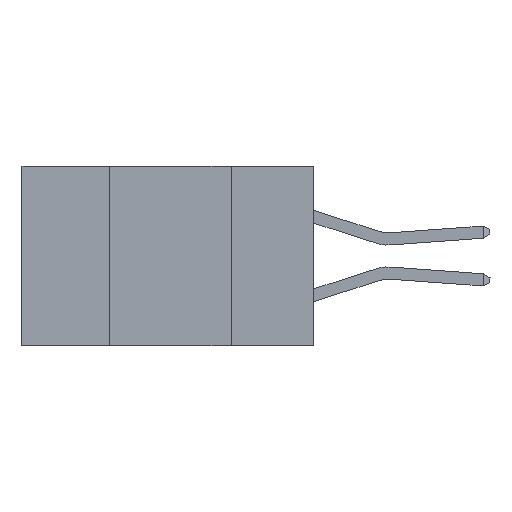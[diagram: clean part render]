
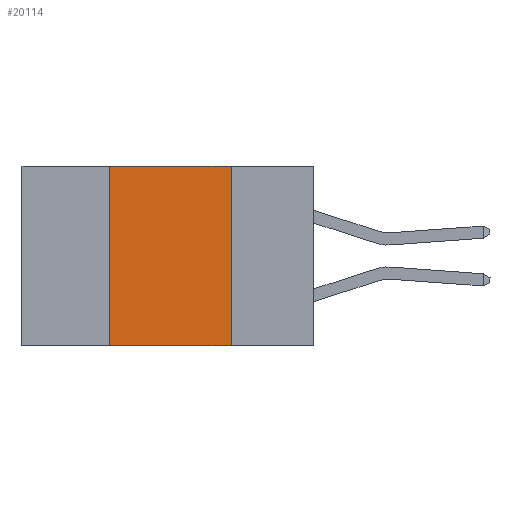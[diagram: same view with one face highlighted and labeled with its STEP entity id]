
A CAD part, left-side view. The second image highlights one B-rep face of the part: STEP entity #20114.
In plain terms, the highlighted planar face has unit normal (-1, 0, 0).
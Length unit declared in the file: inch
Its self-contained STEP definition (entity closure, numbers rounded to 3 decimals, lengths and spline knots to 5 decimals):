
#667 = CARTESIAN_POINT ( 'NONE',  ( 0., 0.17, 0. ) ) ;
#1285 = LINE ( 'NONE', #8244, #15098 ) ;
#1600 = DIRECTION ( 'NONE',  ( 0., 0., 1. ) ) ;
#1718 = ORIENTED_EDGE ( 'NONE', *, *, #7390, .T. ) ;
#2629 = VECTOR ( 'NONE', #1600, 39.37008 ) ;
#2840 = CARTESIAN_POINT ( 'NONE',  ( 0., 0.6, 0. ) ) ;
#3334 = VERTEX_POINT ( 'NONE', #667 ) ;
#4175 = CARTESIAN_POINT ( 'NONE',  ( 0., 0.6, -0.37 ) ) ;
#4380 = FACE_OUTER_BOUND ( 'NONE', #17846, .T. ) ;
#4675 = DIRECTION ( 'NONE',  ( 0., 0., -1. ) ) ;
#5978 = VERTEX_POINT ( 'NONE', #14122 ) ;
#5989 = DIRECTION ( 'NONE',  ( 0., -1., 0. ) ) ;
#6686 = CARTESIAN_POINT ( 'NONE',  ( 0., 0.6, 0. ) ) ;
#6877 = LINE ( 'NONE', #12383, #2629 ) ;
#7390 = EDGE_CURVE ( 'NONE', #12121, #9694, #13743, .T. ) ;
#7624 = EDGE_CURVE ( 'NONE', #5978, #3334, #13443, .T. ) ;
#8244 = CARTESIAN_POINT ( 'NONE',  ( 0., 0.17, 0. ) ) ;
#8831 = CARTESIAN_POINT ( 'NONE',  ( 0., 0.42, -0.37 ) ) ;
#8970 = VECTOR ( 'NONE', #5989, 39.37008 ) ;
#9694 = VERTEX_POINT ( 'NONE', #17954 ) ;
#9961 = PLANE ( 'NONE',  #11155 ) ;
#10014 = DIRECTION ( 'NONE',  ( 0., 0., -1. ) ) ;
#10118 = ORIENTED_EDGE ( 'NONE', *, *, #15347, .F. ) ;
#11155 = AXIS2_PLACEMENT_3D ( 'NONE', #2840, #15417, #4675 ) ;
#11161 = ORIENTED_EDGE ( 'NONE', *, *, #7624, .F. ) ;
#12121 = VERTEX_POINT ( 'NONE', #8831 ) ;
#12383 = CARTESIAN_POINT ( 'NONE',  ( 0., 0.42, 0. ) ) ;
#12884 = VECTOR ( 'NONE', #22623, 39.37008 ) ;
#13443 = LINE ( 'NONE', #6686, #12884 ) ;
#13743 = LINE ( 'NONE', #4175, #8970 ) ;
#14122 = CARTESIAN_POINT ( 'NONE',  ( 0., 0.42, 0. ) ) ;
#15098 = VECTOR ( 'NONE', #10014, 39.37008 ) ;
#15347 = EDGE_CURVE ( 'NONE', #3334, #9694, #1285, .T. ) ;
#15417 = DIRECTION ( 'NONE',  ( 1., 0., 0. ) ) ;
#17846 = EDGE_LOOP ( 'NONE', ( #10118, #11161, #22005, #1718 ) ) ;
#17954 = CARTESIAN_POINT ( 'NONE',  ( 0., 0.17, -0.37 ) ) ;
#20114 = ADVANCED_FACE ( 'NONE', ( #4380 ), #9961, .F. ) ;
#21682 = EDGE_CURVE ( 'NONE', #12121, #5978, #6877, .T. ) ;
#22005 = ORIENTED_EDGE ( 'NONE', *, *, #21682, .F. ) ;
#22623 = DIRECTION ( 'NONE',  ( 0., -1., 0. ) ) ;
